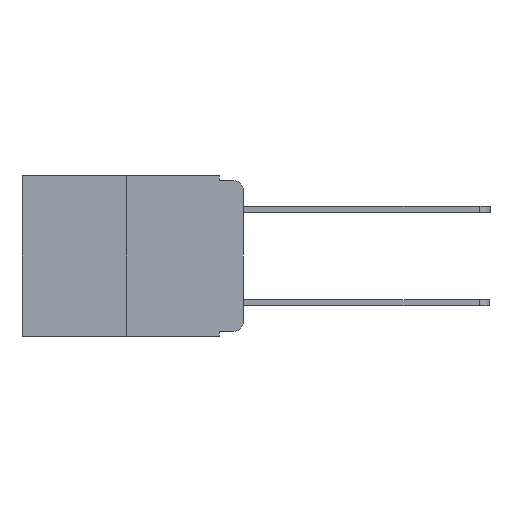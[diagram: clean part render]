
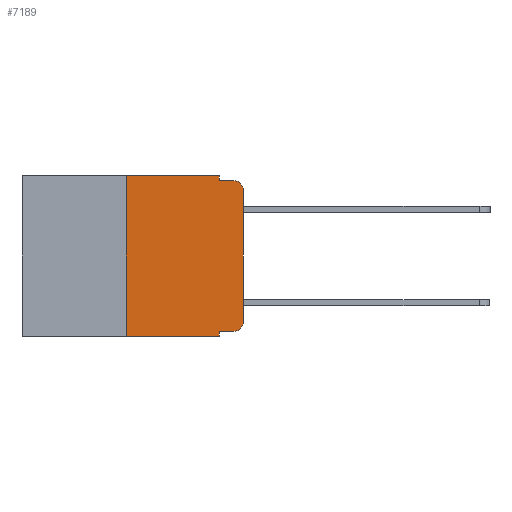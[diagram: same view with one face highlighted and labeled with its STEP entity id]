
A CAD part, left-side view. The second image highlights one B-rep face of the part: STEP entity #7189.
In plain terms, the highlighted planar face has unit normal (-1, 0, 0).
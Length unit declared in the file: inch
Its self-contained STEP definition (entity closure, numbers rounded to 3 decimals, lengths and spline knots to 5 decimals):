
#11 = DIRECTION ( 'NONE',  ( 0., 0., -1. ) ) ;
#495 = VERTEX_POINT ( 'NONE', #13364 ) ;
#609 = DIRECTION ( 'NONE',  ( 0., 0., 1. ) ) ;
#737 = VECTOR ( 'NONE', #16308, 39.37008 ) ;
#807 = DIRECTION ( 'NONE',  ( 0., 0., -1. ) ) ;
#826 = CARTESIAN_POINT ( 'NONE',  ( 0., 0.473, -0.343 ) ) ;
#902 = EDGE_CURVE ( 'NONE', #7987, #2473, #13887, .T. ) ;
#1045 = ORIENTED_EDGE ( 'NONE', *, *, #902, .T. ) ;
#1123 = CARTESIAN_POINT ( 'NONE',  ( 0., 0.051, -0.01 ) ) ;
#1257 = CARTESIAN_POINT ( 'NONE',  ( 0., 0.051, -0.333 ) ) ;
#1408 = CARTESIAN_POINT ( 'NONE',  ( 0., 0.051, 0. ) ) ;
#1536 = DIRECTION ( 'NONE',  ( -1., 0., 0. ) ) ;
#1739 = CARTESIAN_POINT ( 'NONE',  ( 0., 0.473, 0. ) ) ;
#1953 = CARTESIAN_POINT ( 'NONE',  ( 0., 0., -0.313 ) ) ;
#2134 = ORIENTED_EDGE ( 'NONE', *, *, #15778, .F. ) ;
#2473 = VERTEX_POINT ( 'NONE', #11604 ) ;
#2822 = CARTESIAN_POINT ( 'NONE',  ( 0., 0., -0.03 ) ) ;
#2975 = VECTOR ( 'NONE', #609, 39.37008 ) ;
#3202 = ORIENTED_EDGE ( 'NONE', *, *, #14850, .T. ) ;
#3484 = VECTOR ( 'NONE', #16854, 39.37008 ) ;
#3616 = CARTESIAN_POINT ( 'NONE',  ( 0., 0.02, -0.03 ) ) ;
#4457 = LINE ( 'NONE', #1257, #737 ) ;
#4557 = DIRECTION ( 'NONE',  ( 0., 0., -1. ) ) ;
#4722 = AXIS2_PLACEMENT_3D ( 'NONE', #1739, #12754, #4557 ) ;
#4841 = VECTOR ( 'NONE', #10467, 39.37008 ) ;
#5214 = VECTOR ( 'NONE', #11, 39.37008 ) ;
#5267 = VERTEX_POINT ( 'NONE', #5868 ) ;
#5363 = DIRECTION ( 'NONE',  ( 0., -1., 0. ) ) ;
#5645 = ORIENTED_EDGE ( 'NONE', *, *, #17469, .F. ) ;
#5650 = DIRECTION ( 'NONE',  ( 0., 0., -1. ) ) ;
#5868 = CARTESIAN_POINT ( 'NONE',  ( 0., 0.25, -0.343 ) ) ;
#5898 = CARTESIAN_POINT ( 'NONE',  ( 0., 0.051, -0.333 ) ) ;
#6022 = EDGE_CURVE ( 'NONE', #7589, #2473, #13068, .T. ) ;
#6057 = LINE ( 'NONE', #13546, #9712 ) ;
#6117 = DIRECTION ( 'NONE',  ( -1., 0., 0. ) ) ;
#6295 = ORIENTED_EDGE ( 'NONE', *, *, #7641, .T. ) ;
#6613 = CARTESIAN_POINT ( 'NONE',  ( 0., 0.02, -0.333 ) ) ;
#7038 = CARTESIAN_POINT ( 'NONE',  ( 0., 0.051, -0.343 ) ) ;
#7189 = ADVANCED_FACE ( 'NONE', ( #11333 ), #11387, .F. ) ;
#7329 = CARTESIAN_POINT ( 'NONE',  ( 0., 0.25, 0. ) ) ;
#7585 = CARTESIAN_POINT ( 'NONE',  ( 0., 0.051, -0.01 ) ) ;
#7589 = VERTEX_POINT ( 'NONE', #1123 ) ;
#7641 = EDGE_CURVE ( 'NONE', #9360, #17289, #4457, .T. ) ;
#7987 = VERTEX_POINT ( 'NONE', #2822 ) ;
#8224 = VERTEX_POINT ( 'NONE', #1953 ) ;
#8323 = ORIENTED_EDGE ( 'NONE', *, *, #11866, .T. ) ;
#8577 = VERTEX_POINT ( 'NONE', #12408 ) ;
#8966 = DIRECTION ( 'NONE',  ( 0., -1., 0. ) ) ;
#9360 = VERTEX_POINT ( 'NONE', #5898 ) ;
#9486 = CIRCLE ( 'NONE', #11482, 0.02 ) ;
#9712 = VECTOR ( 'NONE', #5363, 39.37008 ) ;
#9870 = EDGE_CURVE ( 'NONE', #8577, #7589, #12497, .T. ) ;
#10023 = AXIS2_PLACEMENT_3D ( 'NONE', #3616, #1536, #807 ) ;
#10273 = LINE ( 'NONE', #14377, #2975 ) ;
#10467 = DIRECTION ( 'NONE',  ( 0., -1., 0. ) ) ;
#11333 = FACE_OUTER_BOUND ( 'NONE', #11998, .T. ) ;
#11387 = PLANE ( 'NONE',  #4722 ) ;
#11482 = AXIS2_PLACEMENT_3D ( 'NONE', #14301, #6117, #15683 ) ;
#11604 = CARTESIAN_POINT ( 'NONE',  ( 0., 0.02, -0.01 ) ) ;
#11866 = EDGE_CURVE ( 'NONE', #8224, #7987, #10273, .T. ) ;
#11998 = EDGE_LOOP ( 'NONE', ( #8323, #1045, #16023, #16214, #16755, #5645, #3202, #2134, #6295, #17679 ) ) ;
#12408 = CARTESIAN_POINT ( 'NONE',  ( 0., 0.051, 0. ) ) ;
#12484 = CARTESIAN_POINT ( 'NONE',  ( 0., 0.051, 0. ) ) ;
#12497 = LINE ( 'NONE', #1408, #5214 ) ;
#12754 = DIRECTION ( 'NONE',  ( 1., 0., 0. ) ) ;
#13068 = LINE ( 'NONE', #7585, #16252 ) ;
#13364 = CARTESIAN_POINT ( 'NONE',  ( 0., 0.25, 0. ) ) ;
#13374 = VECTOR ( 'NONE', #5650, 39.37008 ) ;
#13546 = CARTESIAN_POINT ( 'NONE',  ( 0., 0.473, 0. ) ) ;
#13887 = CIRCLE ( 'NONE', #10023, 0.02 ) ;
#14301 = CARTESIAN_POINT ( 'NONE',  ( 0., 0.02, -0.313 ) ) ;
#14377 = CARTESIAN_POINT ( 'NONE',  ( 0., 0., 0. ) ) ;
#14393 = LINE ( 'NONE', #7329, #3484 ) ;
#14850 = EDGE_CURVE ( 'NONE', #5267, #15186, #15321, .T. ) ;
#15186 = VERTEX_POINT ( 'NONE', #7038 ) ;
#15321 = LINE ( 'NONE', #826, #4841 ) ;
#15683 = DIRECTION ( 'NONE',  ( 0., 0., -1. ) ) ;
#15778 = EDGE_CURVE ( 'NONE', #9360, #15186, #16979, .T. ) ;
#16023 = ORIENTED_EDGE ( 'NONE', *, *, #6022, .F. ) ;
#16214 = ORIENTED_EDGE ( 'NONE', *, *, #9870, .F. ) ;
#16252 = VECTOR ( 'NONE', #8966, 39.37008 ) ;
#16308 = DIRECTION ( 'NONE',  ( 0., -1., 0. ) ) ;
#16755 = ORIENTED_EDGE ( 'NONE', *, *, #17302, .F. ) ;
#16854 = DIRECTION ( 'NONE',  ( 0., 0., 1. ) ) ;
#16979 = LINE ( 'NONE', #12484, #13374 ) ;
#17289 = VERTEX_POINT ( 'NONE', #6613 ) ;
#17302 = EDGE_CURVE ( 'NONE', #495, #8577, #6057, .T. ) ;
#17469 = EDGE_CURVE ( 'NONE', #5267, #495, #14393, .T. ) ;
#17552 = EDGE_CURVE ( 'NONE', #17289, #8224, #9486, .T. ) ;
#17679 = ORIENTED_EDGE ( 'NONE', *, *, #17552, .T. ) ;
